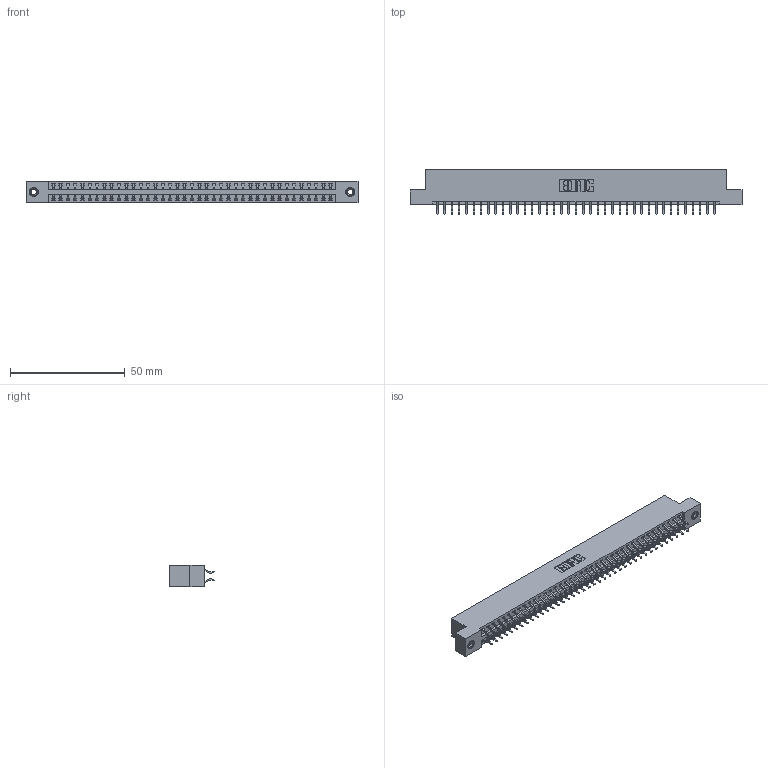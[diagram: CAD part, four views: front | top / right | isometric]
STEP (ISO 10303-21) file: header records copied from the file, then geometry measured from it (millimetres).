
FILE_DESCRIPTION (( 'STEP AP203' ), '1' );
FILE_NAME ('346-078-556-207.STEP', '2018-08-29T06:15:34', ( '' ), ( '' ), 'SwSTEP 2.0', 'SolidWorks 2016', '' );
FILE_SCHEMA (( 'CONFIG_CONTROL_DESIGN' ));
Length unit declared in the file: inch
Products named in the file (4): 345-292-001_556 Tail; 345-250-001_345-250-005-103; 346-078-556-207; 346 Part_Flush Mounting Lugs - 0.156 Dia-TI
Assembly tree (81 placements, depth 2):
  346-078-556-207
    346 Part_Flush Mounting Lugs - 0.156 Dia-TI
    345-292-001_556 Tail  x78
    345-250-001_345-250-005-103  x2
Bounding box: 144.4 x 19.57 x 9.4 mm (x, y, z)
Volume: 14040.8 mm3; surface area: 19214.2 mm2
Topology: 81 solids, 81 shells, 4706 faces, 13959 edges, 9194 vertices
Faces by surface type: plane 3150, cylinder 1540, cone 12, torus 4
Entity records: 27262 total; most frequent: CARTESIAN_POINT 4495, ORIENTED_EDGE 4410, DIRECTION 4027, EDGE_CURVE 2205, VECTOR 1889, LINE 1889, VERTEX_POINT 1464, AXIS2_PLACEMENT_3D 1069
